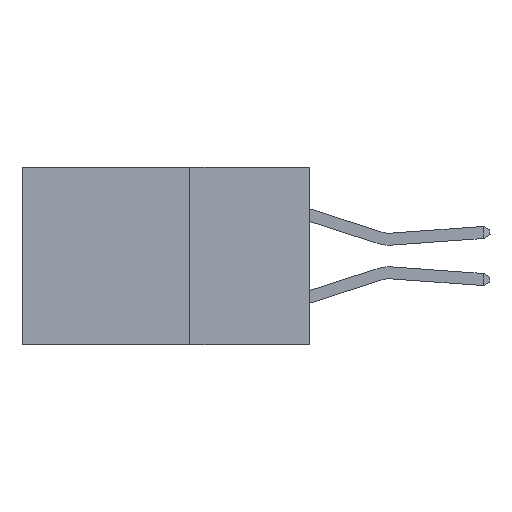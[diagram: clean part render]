
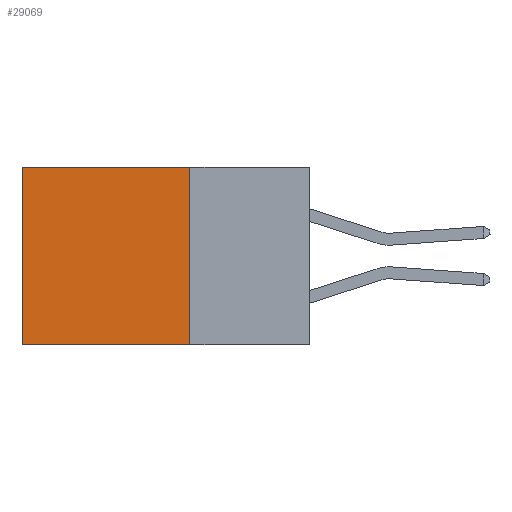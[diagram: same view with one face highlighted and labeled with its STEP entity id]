
A CAD part, left-side view. The second image highlights one B-rep face of the part: STEP entity #29069.
In plain terms, the highlighted planar face has unit normal (-1, 0, 0).
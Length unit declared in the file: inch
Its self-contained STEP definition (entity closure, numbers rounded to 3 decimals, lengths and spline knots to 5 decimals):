
#307 = VERTEX_POINT ( 'NONE', #25615 ) ;
#800 = CARTESIAN_POINT ( 'NONE',  ( 0.298, 0.25, -0.37 ) ) ;
#1341 = LINE ( 'NONE', #9656, #24034 ) ;
#2229 = ORIENTED_EDGE ( 'NONE', *, *, #30011, .F. ) ;
#2620 = DIRECTION ( 'NONE',  ( 0., 1., 0. ) ) ;
#4818 = CARTESIAN_POINT ( 'NONE',  ( 0.298, 0.25, 0. ) ) ;
#4997 = LINE ( 'NONE', #4818, #22155 ) ;
#7176 = PLANE ( 'NONE',  #28588 ) ;
#8381 = LINE ( 'NONE', #29622, #28063 ) ;
#8978 = LINE ( 'NONE', #27711, #17617 ) ;
#9047 = VERTEX_POINT ( 'NONE', #10104 ) ;
#9544 = CARTESIAN_POINT ( 'NONE',  ( 0.298, 0.25, 0. ) ) ;
#9656 = CARTESIAN_POINT ( 'NONE',  ( 0.298, 0.25, -0.37 ) ) ;
#10104 = CARTESIAN_POINT ( 'NONE',  ( 0.298, 0.25, 0. ) ) ;
#10373 = VERTEX_POINT ( 'NONE', #18685 ) ;
#12718 = EDGE_CURVE ( 'NONE', #307, #10373, #8381, .T. ) ;
#14397 = EDGE_CURVE ( 'NONE', #9047, #307, #8978, .T. ) ;
#15303 = EDGE_LOOP ( 'NONE', ( #23649, #22530, #2229, #20851 ) ) ;
#16738 = DIRECTION ( 'NONE',  ( 0., 0., -1. ) ) ;
#17617 = VECTOR ( 'NONE', #27492, 39.37008 ) ;
#18685 = CARTESIAN_POINT ( 'NONE',  ( 0.298, 0.6, -0.37 ) ) ;
#20495 = DIRECTION ( 'NONE',  ( 0., 0., -1. ) ) ;
#20698 = FACE_OUTER_BOUND ( 'NONE', #15303, .T. ) ;
#20851 = ORIENTED_EDGE ( 'NONE', *, *, #14397, .T. ) ;
#21409 = EDGE_CURVE ( 'NONE', #29577, #10373, #1341, .T. ) ;
#22155 = VECTOR ( 'NONE', #28297, 39.37008 ) ;
#22530 = ORIENTED_EDGE ( 'NONE', *, *, #21409, .F. ) ;
#23649 = ORIENTED_EDGE ( 'NONE', *, *, #12718, .T. ) ;
#24034 = VECTOR ( 'NONE', #2620, 39.37008 ) ;
#25615 = CARTESIAN_POINT ( 'NONE',  ( 0.298, 0.6, 0. ) ) ;
#26250 = DIRECTION ( 'NONE',  ( 1., 0., 0. ) ) ;
#27492 = DIRECTION ( 'NONE',  ( 0., 1., 0. ) ) ;
#27711 = CARTESIAN_POINT ( 'NONE',  ( 0.298, 0.25, 0. ) ) ;
#28063 = VECTOR ( 'NONE', #20495, 39.37008 ) ;
#28297 = DIRECTION ( 'NONE',  ( 0., 0., -1. ) ) ;
#28588 = AXIS2_PLACEMENT_3D ( 'NONE', #9544, #26250, #16738 ) ;
#29069 = ADVANCED_FACE ( 'NONE', ( #20698 ), #7176, .F. ) ;
#29577 = VERTEX_POINT ( 'NONE', #800 ) ;
#29622 = CARTESIAN_POINT ( 'NONE',  ( 0.298, 0.6, 0. ) ) ;
#30011 = EDGE_CURVE ( 'NONE', #9047, #29577, #4997, .T. ) ;
